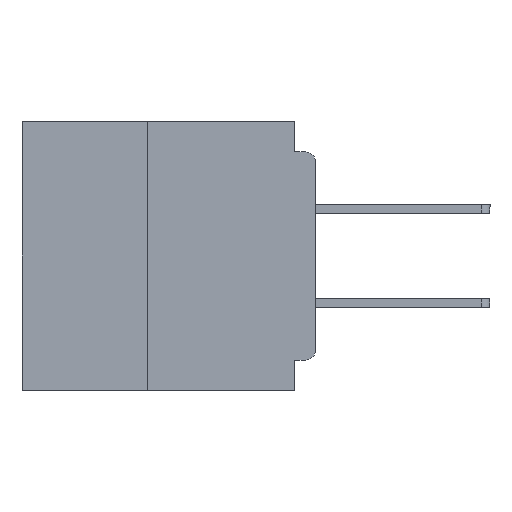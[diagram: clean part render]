
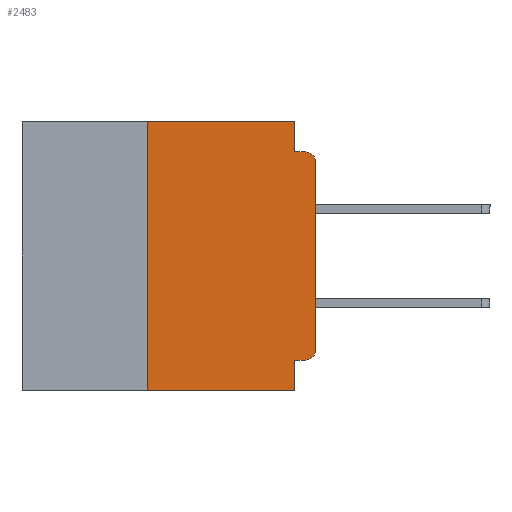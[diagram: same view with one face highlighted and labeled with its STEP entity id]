
A CAD part, left-side view. The second image highlights one B-rep face of the part: STEP entity #2483.
In plain terms, the highlighted planar face has unit normal (-1, 0, 0).
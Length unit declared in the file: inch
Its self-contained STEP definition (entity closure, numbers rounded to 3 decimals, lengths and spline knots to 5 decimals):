
#851 = VECTOR ( 'NONE', #54109, 39.37008 ) ;
#1239 = DIRECTION ( 'NONE',  ( -1., 0., 0. ) ) ;
#1336 = CARTESIAN_POINT ( 'NONE',  ( 0., 0.25, -0.4 ) ) ;
#1489 = LINE ( 'NONE', #17641, #46385 ) ;
#2042 = EDGE_CURVE ( 'NONE', #34498, #45071, #26198, .T. ) ;
#2483 = ADVANCED_FACE ( 'NONE', ( #37672 ), #50551, .F. ) ;
#3015 = VECTOR ( 'NONE', #53950, 39.37008 ) ;
#5417 = EDGE_CURVE ( 'NONE', #49635, #45869, #1489, .T. ) ;
#6384 = ORIENTED_EDGE ( 'NONE', *, *, #25622, .F. ) ;
#6598 = EDGE_CURVE ( 'NONE', #42316, #23329, #19772, .T. ) ;
#7379 = DIRECTION ( 'NONE',  ( 0., 1., 0. ) ) ;
#10114 = CARTESIAN_POINT ( 'NONE',  ( 0., 0.031, -0.4 ) ) ;
#10613 = EDGE_LOOP ( 'NONE', ( #38343, #33623, #34969, #49198, #50546, #43121, #34322, #25463, #6384, #52573 ) ) ;
#10626 = DIRECTION ( 'NONE',  ( 0., 0., -1. ) ) ;
#10761 = CARTESIAN_POINT ( 'NONE',  ( 0., 0.015, -0.34 ) ) ;
#11577 = EDGE_CURVE ( 'NONE', #34299, #49635, #15390, .T. ) ;
#12437 = LINE ( 'NONE', #41135, #851 ) ;
#12811 = CARTESIAN_POINT ( 'NONE',  ( 0., 0.031, -0.4 ) ) ;
#13139 = AXIS2_PLACEMENT_3D ( 'NONE', #10761, #41197, #15126 ) ;
#13974 = CARTESIAN_POINT ( 'NONE',  ( 0., 0.031, -0.355 ) ) ;
#14449 = CARTESIAN_POINT ( 'NONE',  ( 0., 0., -0.06 ) ) ;
#14575 = VECTOR ( 'NONE', #10626, 39.37008 ) ;
#14914 = CARTESIAN_POINT ( 'NONE',  ( 0., 0.437, -0.4 ) ) ;
#15126 = DIRECTION ( 'NONE',  ( 0., 0., -1. ) ) ;
#15390 = LINE ( 'NONE', #1336, #35826 ) ;
#16817 = LINE ( 'NONE', #36632, #18188 ) ;
#17252 = EDGE_CURVE ( 'NONE', #45869, #37673, #12437, .T. ) ;
#17489 = DIRECTION ( 'NONE',  ( 0., -1., 0. ) ) ;
#17641 = CARTESIAN_POINT ( 'NONE',  ( 0., 0.437, 0. ) ) ;
#18188 = VECTOR ( 'NONE', #23692, 39.37008 ) ;
#19772 = CIRCLE ( 'NONE', #55125, 0.015 ) ;
#20619 = DIRECTION ( 'NONE',  ( 0., 0., 1. ) ) ;
#20704 = CARTESIAN_POINT ( 'NONE',  ( 0., 0.031, -0.045 ) ) ;
#23329 = VERTEX_POINT ( 'NONE', #46622 ) ;
#23692 = DIRECTION ( 'NONE',  ( 0., -1., 0. ) ) ;
#25200 = CARTESIAN_POINT ( 'NONE',  ( 0., 0.25, 0. ) ) ;
#25463 = ORIENTED_EDGE ( 'NONE', *, *, #2042, .F. ) ;
#25622 = EDGE_CURVE ( 'NONE', #44804, #34498, #41351, .T. ) ;
#26140 = EDGE_CURVE ( 'NONE', #37673, #23329, #16817, .T. ) ;
#26198 = LINE ( 'NONE', #10114, #14575 ) ;
#27002 = CIRCLE ( 'NONE', #13139, 0.015 ) ;
#27292 = EDGE_CURVE ( 'NONE', #34299, #45071, #37750, .T. ) ;
#27369 = CARTESIAN_POINT ( 'NONE',  ( 0., 0.015, -0.06 ) ) ;
#28648 = VECTOR ( 'NONE', #20619, 39.37008 ) ;
#29848 = VECTOR ( 'NONE', #7379, 39.37008 ) ;
#30023 = LINE ( 'NONE', #33599, #28648 ) ;
#31385 = CARTESIAN_POINT ( 'NONE',  ( 0., 0., -0.34 ) ) ;
#31749 = DIRECTION ( 'NONE',  ( 0., 0., -1. ) ) ;
#33487 = CARTESIAN_POINT ( 'NONE',  ( 0., 0., -0.355 ) ) ;
#33599 = CARTESIAN_POINT ( 'NONE',  ( 0., 0., 0. ) ) ;
#33623 = ORIENTED_EDGE ( 'NONE', *, *, #6598, .T. ) ;
#34299 = VERTEX_POINT ( 'NONE', #38172 ) ;
#34322 = ORIENTED_EDGE ( 'NONE', *, *, #27292, .T. ) ;
#34439 = AXIS2_PLACEMENT_3D ( 'NONE', #50364, #49933, #49870 ) ;
#34498 = VERTEX_POINT ( 'NONE', #13974 ) ;
#34969 = ORIENTED_EDGE ( 'NONE', *, *, #26140, .F. ) ;
#35826 = VECTOR ( 'NONE', #44684, 39.37008 ) ;
#36632 = CARTESIAN_POINT ( 'NONE',  ( 0., 0., -0.045 ) ) ;
#36812 = CARTESIAN_POINT ( 'NONE',  ( 0., 0.015, -0.355 ) ) ;
#37672 = FACE_OUTER_BOUND ( 'NONE', #10613, .T. ) ;
#37673 = VERTEX_POINT ( 'NONE', #20704 ) ;
#37750 = LINE ( 'NONE', #14914, #3015 ) ;
#38172 = CARTESIAN_POINT ( 'NONE',  ( 0., 0.25, -0.4 ) ) ;
#38343 = ORIENTED_EDGE ( 'NONE', *, *, #47770, .T. ) ;
#41135 = CARTESIAN_POINT ( 'NONE',  ( 0., 0.031, 0. ) ) ;
#41197 = DIRECTION ( 'NONE',  ( -1., 0., 0. ) ) ;
#41351 = LINE ( 'NONE', #33487, #29848 ) ;
#42316 = VERTEX_POINT ( 'NONE', #14449 ) ;
#43121 = ORIENTED_EDGE ( 'NONE', *, *, #11577, .F. ) ;
#44283 = CARTESIAN_POINT ( 'NONE',  ( 0., 0.031, 0. ) ) ;
#44684 = DIRECTION ( 'NONE',  ( 0., 0., 1. ) ) ;
#44804 = VERTEX_POINT ( 'NONE', #36812 ) ;
#45071 = VERTEX_POINT ( 'NONE', #12811 ) ;
#45869 = VERTEX_POINT ( 'NONE', #44283 ) ;
#46385 = VECTOR ( 'NONE', #17489, 39.37008 ) ;
#46551 = EDGE_CURVE ( 'NONE', #44804, #53281, #27002, .T. ) ;
#46622 = CARTESIAN_POINT ( 'NONE',  ( 0., 0.015, -0.045 ) ) ;
#47770 = EDGE_CURVE ( 'NONE', #53281, #42316, #30023, .T. ) ;
#49198 = ORIENTED_EDGE ( 'NONE', *, *, #17252, .F. ) ;
#49635 = VERTEX_POINT ( 'NONE', #25200 ) ;
#49870 = DIRECTION ( 'NONE',  ( 0., 0., -1. ) ) ;
#49933 = DIRECTION ( 'NONE',  ( 1., 0., 0. ) ) ;
#50364 = CARTESIAN_POINT ( 'NONE',  ( 0., 0.437, 0. ) ) ;
#50546 = ORIENTED_EDGE ( 'NONE', *, *, #5417, .F. ) ;
#50551 = PLANE ( 'NONE',  #34439 ) ;
#52573 = ORIENTED_EDGE ( 'NONE', *, *, #46551, .T. ) ;
#53281 = VERTEX_POINT ( 'NONE', #31385 ) ;
#53950 = DIRECTION ( 'NONE',  ( 0., -1., 0. ) ) ;
#54109 = DIRECTION ( 'NONE',  ( 0., 0., -1. ) ) ;
#55125 = AXIS2_PLACEMENT_3D ( 'NONE', #27369, #1239, #31749 ) ;
